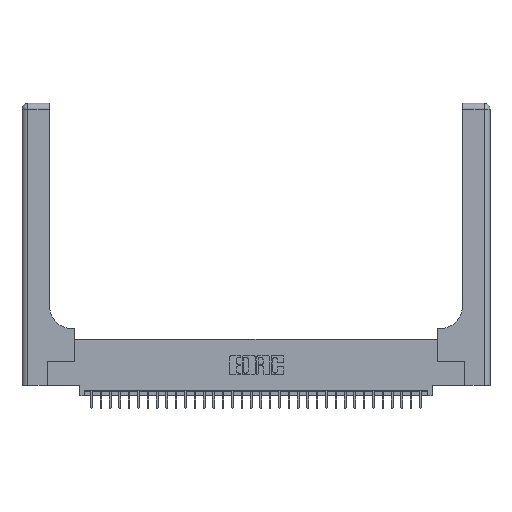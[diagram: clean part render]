
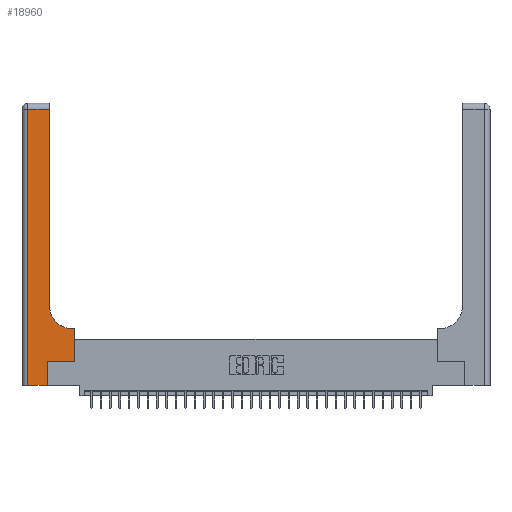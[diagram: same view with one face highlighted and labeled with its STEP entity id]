
A CAD part, top view. The second image highlights one B-rep face of the part: STEP entity #18960.
In plain terms, the highlighted planar face has unit normal (0, 0, 1).
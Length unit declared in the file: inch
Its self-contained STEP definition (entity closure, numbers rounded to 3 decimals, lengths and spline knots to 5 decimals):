
#91 = DIRECTION ( 'NONE',  ( 0., 0., -1. ) ) ;
#131 = VECTOR ( 'NONE', #10040, 39.37008 ) ;
#272 = LINE ( 'NONE', #10921, #7446 ) ;
#586 = EDGE_CURVE ( 'NONE', #17612, #34410, #23311, .T. ) ;
#770 = VERTEX_POINT ( 'NONE', #3578 ) ;
#980 = EDGE_CURVE ( 'NONE', #26772, #15439, #16113, .T. ) ;
#1092 = VERTEX_POINT ( 'NONE', #3695 ) ;
#1541 = CARTESIAN_POINT ( 'NONE',  ( 0.5585, 0.25, 0.37 ) ) ;
#2311 = CARTESIAN_POINT ( 'NONE',  ( 0.2915, 0.6, 0.37 ) ) ;
#2870 = ORIENTED_EDGE ( 'NONE', *, *, #16135, .T. ) ;
#3320 = AXIS2_PLACEMENT_3D ( 'NONE', #14994, #25634, #23008 ) ;
#3578 = CARTESIAN_POINT ( 'NONE',  ( 0.2915, 2.94, 0.37 ) ) ;
#3695 = CARTESIAN_POINT ( 'NONE',  ( 0.06, 0., 0.37 ) ) ;
#4174 = CARTESIAN_POINT ( 'NONE',  ( 0., 0., 0.37 ) ) ;
#4313 = CARTESIAN_POINT ( 'NONE',  ( 0.269, 0.25, 0.37 ) ) ;
#6854 = ORIENTED_EDGE ( 'NONE', *, *, #10981, .T. ) ;
#7423 = EDGE_LOOP ( 'NONE', ( #2870, #10316, #6854, #8243, #14152, #18708, #7884, #23708, #19292 ) ) ;
#7446 = VECTOR ( 'NONE', #21548, 39.37008 ) ;
#7767 = CARTESIAN_POINT ( 'NONE',  ( 0.5415, 0.85, 0.37 ) ) ;
#7806 = VERTEX_POINT ( 'NONE', #10473 ) ;
#7884 = ORIENTED_EDGE ( 'NONE', *, *, #24744, .T. ) ;
#8243 = ORIENTED_EDGE ( 'NONE', *, *, #33154, .T. ) ;
#8359 = CARTESIAN_POINT ( 'NONE',  ( 0.06, 3., 0.37 ) ) ;
#9574 = DIRECTION ( 'NONE',  ( 0., 1., 0. ) ) ;
#10040 = DIRECTION ( 'NONE',  ( 1., 0., 0. ) ) ;
#10316 = ORIENTED_EDGE ( 'NONE', *, *, #16662, .T. ) ;
#10473 = CARTESIAN_POINT ( 'NONE',  ( 0.06, 2.94, 0.37 ) ) ;
#10921 = CARTESIAN_POINT ( 'NONE',  ( 0.2915, 3., 0.37 ) ) ;
#10977 = DIRECTION ( 'NONE',  ( 0., -1., 0. ) ) ;
#10981 = EDGE_CURVE ( 'NONE', #7806, #1092, #32255, .T. ) ;
#11093 = VERTEX_POINT ( 'NONE', #23141 ) ;
#11520 = EDGE_CURVE ( 'NONE', #11093, #17612, #15083, .T. ) ;
#12046 = DIRECTION ( 'NONE',  ( 1., 0., 0. ) ) ;
#12161 = AXIS2_PLACEMENT_3D ( 'NONE', #7767, #91, #28906 ) ;
#13148 = CARTESIAN_POINT ( 'NONE',  ( 0.5585, 0.25, 0.37 ) ) ;
#13635 = DIRECTION ( 'NONE',  ( -1., 0., 0. ) ) ;
#14152 = ORIENTED_EDGE ( 'NONE', *, *, #11520, .T. ) ;
#14394 = CARTESIAN_POINT ( 'NONE',  ( 0.269, 0., 0.37 ) ) ;
#14994 = CARTESIAN_POINT ( 'NONE',  ( 0., 3., 0.37 ) ) ;
#15083 = LINE ( 'NONE', #14394, #19101 ) ;
#15221 = VECTOR ( 'NONE', #34105, 39.37008 ) ;
#15439 = VERTEX_POINT ( 'NONE', #21375 ) ;
#16113 = LINE ( 'NONE', #2311, #15221 ) ;
#16135 = EDGE_CURVE ( 'NONE', #23484, #770, #272, .T. ) ;
#16662 = EDGE_CURVE ( 'NONE', #770, #7806, #34406, .T. ) ;
#17454 = PLANE ( 'NONE',  #3320 ) ;
#17612 = VERTEX_POINT ( 'NONE', #19350 ) ;
#18434 = CARTESIAN_POINT ( 'NONE',  ( 0.5585, 0.6, 0.37 ) ) ;
#18708 = ORIENTED_EDGE ( 'NONE', *, *, #586, .T. ) ;
#18960 = ADVANCED_FACE ( 'NONE', ( #22833 ), #17454, .F. ) ;
#19039 = VECTOR ( 'NONE', #10977, 39.37008 ) ;
#19101 = VECTOR ( 'NONE', #25025, 39.37008 ) ;
#19292 = ORIENTED_EDGE ( 'NONE', *, *, #31086, .T. ) ;
#19350 = CARTESIAN_POINT ( 'NONE',  ( 0.269, 0.25, 0.37 ) ) ;
#19952 = CIRCLE ( 'NONE', #12161, 0.25 ) ;
#20049 = CARTESIAN_POINT ( 'NONE',  ( 0.2915, 0.85, 0.37 ) ) ;
#20393 = LINE ( 'NONE', #4174, #25632 ) ;
#21099 = VECTOR ( 'NONE', #9574, 39.37008 ) ;
#21375 = CARTESIAN_POINT ( 'NONE',  ( 0.5415, 0.6, 0.37 ) ) ;
#21548 = DIRECTION ( 'NONE',  ( 0., 1., 0. ) ) ;
#22833 = FACE_OUTER_BOUND ( 'NONE', #7423, .T. ) ;
#23008 = DIRECTION ( 'NONE',  ( -1., 0., 0. ) ) ;
#23141 = CARTESIAN_POINT ( 'NONE',  ( 0.269, 0., 0.37 ) ) ;
#23311 = LINE ( 'NONE', #4313, #131 ) ;
#23484 = VERTEX_POINT ( 'NONE', #20049 ) ;
#23708 = ORIENTED_EDGE ( 'NONE', *, *, #980, .T. ) ;
#24744 = EDGE_CURVE ( 'NONE', #34410, #26772, #32773, .T. ) ;
#25025 = DIRECTION ( 'NONE',  ( 0., 1., 0. ) ) ;
#25632 = VECTOR ( 'NONE', #12046, 39.37008 ) ;
#25634 = DIRECTION ( 'NONE',  ( 0., 0., -1. ) ) ;
#26772 = VERTEX_POINT ( 'NONE', #18434 ) ;
#28906 = DIRECTION ( 'NONE',  ( 1., 0., 0. ) ) ;
#29728 = VECTOR ( 'NONE', #13635, 39.37008 ) ;
#31086 = EDGE_CURVE ( 'NONE', #15439, #23484, #19952, .T. ) ;
#31944 = CARTESIAN_POINT ( 'NONE',  ( 0., 2.94, 0.37 ) ) ;
#32255 = LINE ( 'NONE', #8359, #19039 ) ;
#32773 = LINE ( 'NONE', #1541, #21099 ) ;
#33154 = EDGE_CURVE ( 'NONE', #1092, #11093, #20393, .T. ) ;
#34105 = DIRECTION ( 'NONE',  ( -1., 0., 0. ) ) ;
#34406 = LINE ( 'NONE', #31944, #29728 ) ;
#34410 = VERTEX_POINT ( 'NONE', #13148 ) ;
